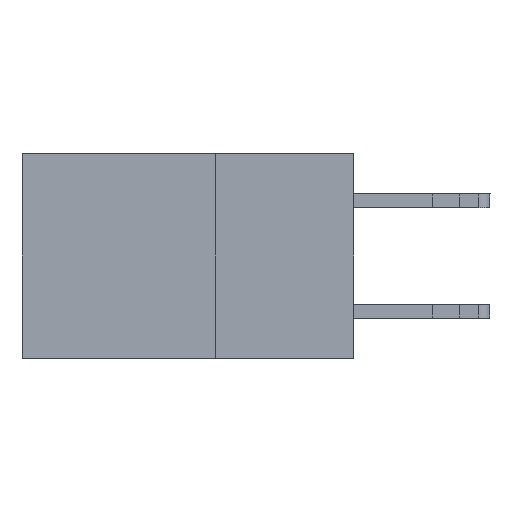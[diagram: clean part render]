
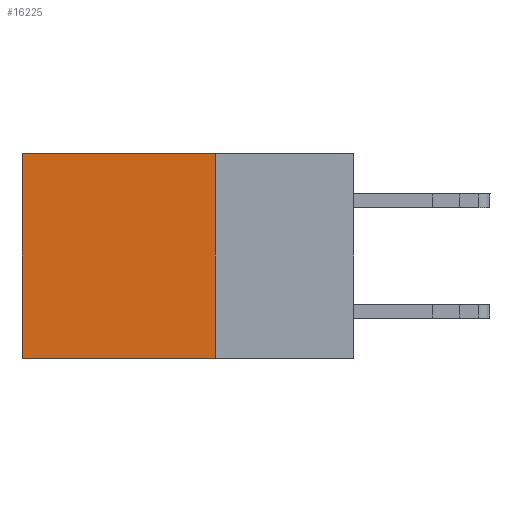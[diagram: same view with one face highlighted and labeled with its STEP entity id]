
A CAD part, left-side view. The second image highlights one B-rep face of the part: STEP entity #16225.
In plain terms, the highlighted planar face has unit normal (-1, 0, 0).
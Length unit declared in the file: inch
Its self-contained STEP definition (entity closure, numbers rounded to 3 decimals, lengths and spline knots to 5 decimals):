
#500 = EDGE_LOOP ( 'NONE', ( #13223, #11631, #17878, #21110 ) ) ;
#1409 = EDGE_CURVE ( 'NONE', #12216, #6020, #4276, .T. ) ;
#2022 = CARTESIAN_POINT ( 'NONE',  ( 0.2875, 0.25, 0. ) ) ;
#2040 = LINE ( 'NONE', #20275, #2907 ) ;
#2406 = CARTESIAN_POINT ( 'NONE',  ( 0.2875, 0.25, -0.37 ) ) ;
#2907 = VECTOR ( 'NONE', #9345, 39.37008 ) ;
#3143 = VECTOR ( 'NONE', #9432, 39.37008 ) ;
#3865 = EDGE_CURVE ( 'NONE', #21483, #16927, #8446, .T. ) ;
#3888 = DIRECTION ( 'NONE',  ( 1., 0., 0. ) ) ;
#4276 = LINE ( 'NONE', #2022, #3143 ) ;
#5327 = CARTESIAN_POINT ( 'NONE',  ( 0.2875, 0.25, -0.37 ) ) ;
#5983 = EDGE_CURVE ( 'NONE', #12216, #21483, #2040, .T. ) ;
#6020 = VERTEX_POINT ( 'NONE', #2406 ) ;
#6240 = EDGE_CURVE ( 'NONE', #6020, #16927, #14892, .T. ) ;
#6290 = PLANE ( 'NONE',  #7158 ) ;
#6872 = VECTOR ( 'NONE', #23624, 39.37008 ) ;
#7158 = AXIS2_PLACEMENT_3D ( 'NONE', #19596, #3888, #14887 ) ;
#7175 = CARTESIAN_POINT ( 'NONE',  ( 0.2875, 0.6, -0.37 ) ) ;
#8446 = LINE ( 'NONE', #20005, #10168 ) ;
#9345 = DIRECTION ( 'NONE',  ( 0., 1., 0. ) ) ;
#9432 = DIRECTION ( 'NONE',  ( 0., 0., -1. ) ) ;
#10168 = VECTOR ( 'NONE', #14527, 39.37008 ) ;
#10688 = FACE_OUTER_BOUND ( 'NONE', #500, .T. ) ;
#11631 = ORIENTED_EDGE ( 'NONE', *, *, #6240, .F. ) ;
#12216 = VERTEX_POINT ( 'NONE', #16824 ) ;
#13223 = ORIENTED_EDGE ( 'NONE', *, *, #3865, .T. ) ;
#14527 = DIRECTION ( 'NONE',  ( 0., 0., -1. ) ) ;
#14887 = DIRECTION ( 'NONE',  ( 0., 0., -1. ) ) ;
#14892 = LINE ( 'NONE', #5327, #6872 ) ;
#16225 = ADVANCED_FACE ( 'NONE', ( #10688 ), #6290, .F. ) ;
#16824 = CARTESIAN_POINT ( 'NONE',  ( 0.2875, 0.25, 0. ) ) ;
#16927 = VERTEX_POINT ( 'NONE', #7175 ) ;
#17878 = ORIENTED_EDGE ( 'NONE', *, *, #1409, .F. ) ;
#19596 = CARTESIAN_POINT ( 'NONE',  ( 0.2875, 0.25, 0. ) ) ;
#20005 = CARTESIAN_POINT ( 'NONE',  ( 0.2875, 0.6, 0. ) ) ;
#20275 = CARTESIAN_POINT ( 'NONE',  ( 0.2875, 0.25, 0. ) ) ;
#20591 = CARTESIAN_POINT ( 'NONE',  ( 0.2875, 0.6, 0. ) ) ;
#21110 = ORIENTED_EDGE ( 'NONE', *, *, #5983, .T. ) ;
#21483 = VERTEX_POINT ( 'NONE', #20591 ) ;
#23624 = DIRECTION ( 'NONE',  ( 0., 1., 0. ) ) ;
